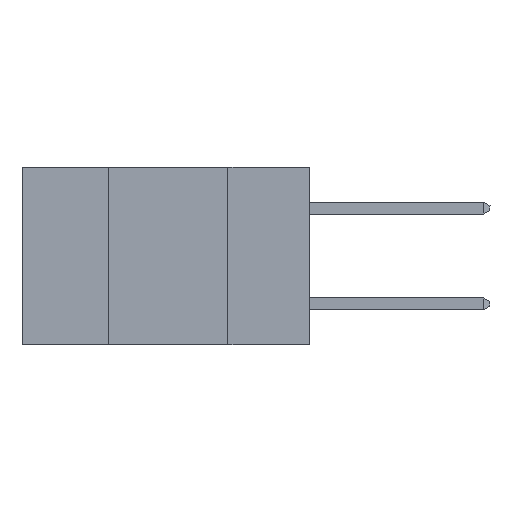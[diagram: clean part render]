
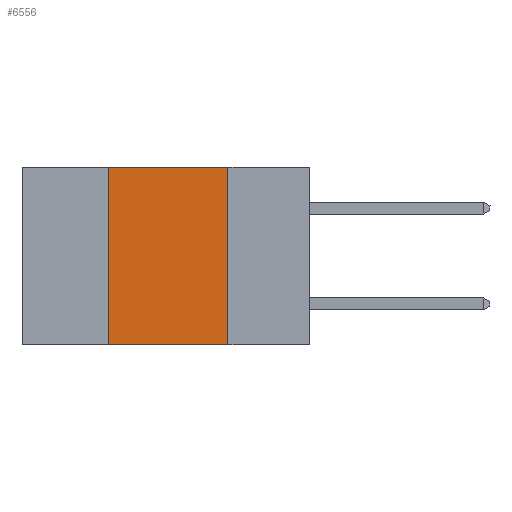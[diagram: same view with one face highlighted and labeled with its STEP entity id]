
A CAD part, left-side view. The second image highlights one B-rep face of the part: STEP entity #6556.
In plain terms, the highlighted planar face has unit normal (-1, 0, 0).
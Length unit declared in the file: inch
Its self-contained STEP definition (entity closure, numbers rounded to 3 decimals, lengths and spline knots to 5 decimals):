
#101 = CARTESIAN_POINT ( 'NONE',  ( 0., 0.42, -0.37 ) ) ;
#406 = CARTESIAN_POINT ( 'NONE',  ( 0., 0.17, 0. ) ) ;
#762 = CARTESIAN_POINT ( 'NONE',  ( 0., 0.42, 0. ) ) ;
#1292 = VERTEX_POINT ( 'NONE', #2377 ) ;
#1329 = DIRECTION ( 'NONE',  ( 0., 0., -1. ) ) ;
#1333 = AXIS2_PLACEMENT_3D ( 'NONE', #6017, #3399, #9578 ) ;
#1353 = CARTESIAN_POINT ( 'NONE',  ( 0., 0.6, -0.37 ) ) ;
#1368 = CARTESIAN_POINT ( 'NONE',  ( 0., 0.17, 0. ) ) ;
#1841 = CARTESIAN_POINT ( 'NONE',  ( 0., 0.17, -0.37 ) ) ;
#2377 = CARTESIAN_POINT ( 'NONE',  ( 0., 0.42, 0. ) ) ;
#2430 = VECTOR ( 'NONE', #7035, 39.37008 ) ;
#2473 = PLANE ( 'NONE',  #1333 ) ;
#3399 = DIRECTION ( 'NONE',  ( 1., 0., 0. ) ) ;
#3482 = VECTOR ( 'NONE', #4081, 39.37008 ) ;
#4081 = DIRECTION ( 'NONE',  ( 0., -1., 0. ) ) ;
#5752 = FACE_OUTER_BOUND ( 'NONE', #10181, .T. ) ;
#5832 = LINE ( 'NONE', #1353, #3482 ) ;
#6017 = CARTESIAN_POINT ( 'NONE',  ( 0., 0.6, 0. ) ) ;
#6556 = ADVANCED_FACE ( 'NONE', ( #5752 ), #2473, .F. ) ;
#6711 = VERTEX_POINT ( 'NONE', #1841 ) ;
#6752 = LINE ( 'NONE', #8346, #11121 ) ;
#7035 = DIRECTION ( 'NONE',  ( 0., 0., 1. ) ) ;
#7264 = VERTEX_POINT ( 'NONE', #1368 ) ;
#7641 = EDGE_CURVE ( 'NONE', #8769, #6711, #5832, .T. ) ;
#8009 = VECTOR ( 'NONE', #1329, 39.37008 ) ;
#8346 = CARTESIAN_POINT ( 'NONE',  ( 0., 0.6, 0. ) ) ;
#8554 = LINE ( 'NONE', #406, #8009 ) ;
#8769 = VERTEX_POINT ( 'NONE', #101 ) ;
#9578 = DIRECTION ( 'NONE',  ( 0., 0., -1. ) ) ;
#9772 = LINE ( 'NONE', #762, #2430 ) ;
#10181 = EDGE_LOOP ( 'NONE', ( #10405, #10456, #10507, #10532 ) ) ;
#10405 = ORIENTED_EDGE ( 'NONE', *, *, #11385, .F. ) ;
#10456 = ORIENTED_EDGE ( 'NONE', *, *, #11302, .F. ) ;
#10507 = ORIENTED_EDGE ( 'NONE', *, *, #10719, .F. ) ;
#10532 = ORIENTED_EDGE ( 'NONE', *, *, #7641, .T. ) ;
#10719 = EDGE_CURVE ( 'NONE', #8769, #1292, #9772, .T. ) ;
#10966 = DIRECTION ( 'NONE',  ( 0., -1., 0. ) ) ;
#11121 = VECTOR ( 'NONE', #10966, 39.37008 ) ;
#11302 = EDGE_CURVE ( 'NONE', #1292, #7264, #6752, .T. ) ;
#11385 = EDGE_CURVE ( 'NONE', #7264, #6711, #8554, .T. ) ;
